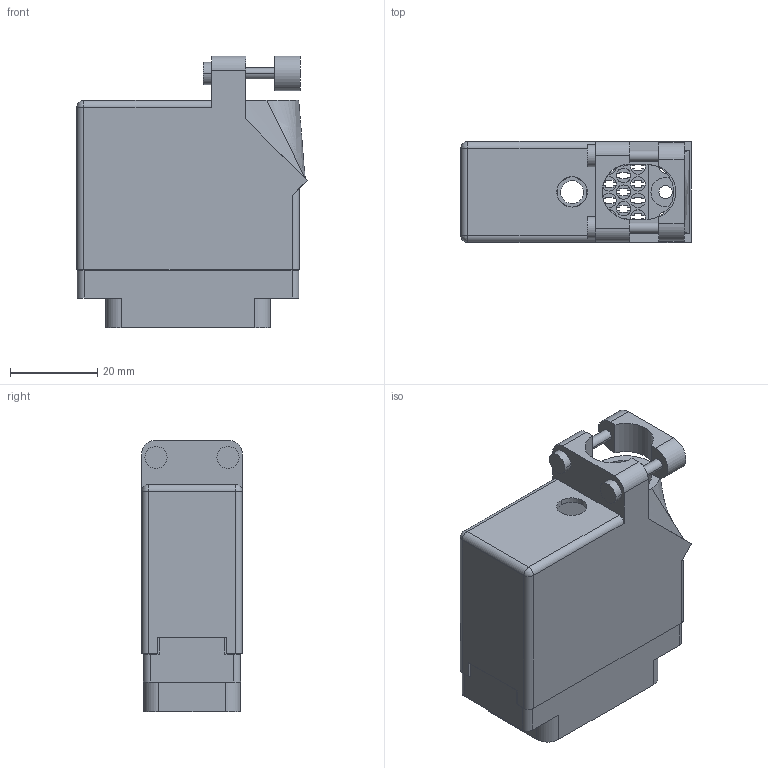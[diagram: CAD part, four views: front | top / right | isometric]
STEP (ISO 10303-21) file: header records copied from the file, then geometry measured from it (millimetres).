
FILE_DESCRIPTION (( 'STEP AP203' ), '1' );
FILE_NAME ('516-038-000-310.STEP', '2020-03-09T18:12:37', ( '' ), ( '' ), 'SwSTEP 2.0', 'SolidWorks 2016', '' );
FILE_SCHEMA (( 'CONFIG_CONTROL_DESIGN' ));
Length unit declared in the file: inch
Products named in the file (3): 516 Plug Insulator_038; 516-038-000-310; 516-230-001_Plastic - 038 Top Entry
Assembly tree (2 placements, depth 2):
  516-038-000-310
    516 Plug Insulator_038
    516-230-001_Plastic - 038 Top Entry
Bounding box: 52.85 x 23.11 x 62.28 mm (x, y, z)
Volume: 19260.9 mm3; surface area: 25483.2 mm2
Topology: 2 solids, 2 shells, 957 faces, 2788 edges, 1854 vertices
Faces by surface type: plane 678, cylinder 272, bspline 3, cone 2, sphere 2
Entity records: 32190 total; most frequent: CARTESIAN_POINT 5695, ORIENTED_EDGE 5572, DIRECTION 5395, EDGE_CURVE 2786, VECTOR 2087, LINE 2087, VERTEX_POINT 1854, AXIS2_PLACEMENT_3D 1654
